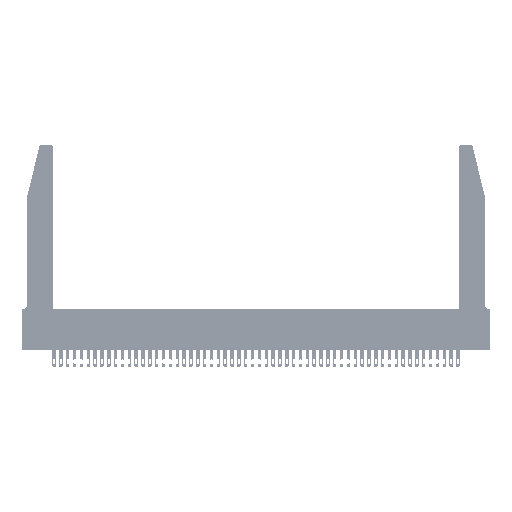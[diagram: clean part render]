
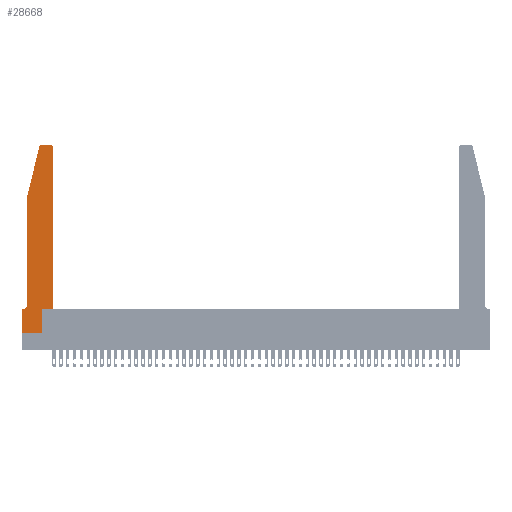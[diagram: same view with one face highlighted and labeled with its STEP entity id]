
A CAD part, top view. The second image highlights one B-rep face of the part: STEP entity #28668.
In plain terms, the highlighted planar face has unit normal (0, 0, 1).
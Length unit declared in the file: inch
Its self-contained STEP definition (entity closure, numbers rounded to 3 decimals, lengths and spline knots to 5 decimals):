
#95 = VERTEX_POINT ( 'NONE', #23272 ) ;
#1008 = EDGE_CURVE ( 'NONE', #95, #37372, #23729, .T. ) ;
#2778 = VERTEX_POINT ( 'NONE', #43819 ) ;
#3142 = LINE ( 'NONE', #47162, #42280 ) ;
#3506 = LINE ( 'NONE', #4900, #23275 ) ;
#3687 = CARTESIAN_POINT ( 'NONE',  ( 0.2605, 2.75, 0.37 ) ) ;
#4401 = AXIS2_PLACEMENT_3D ( 'NONE', #20127, #46738, #35255 ) ;
#4447 = EDGE_CURVE ( 'NONE', #40174, #19119, #18785, .T. ) ;
#4479 = DIRECTION ( 'NONE',  ( 0., 1., 0. ) ) ;
#4484 = DIRECTION ( 'NONE',  ( 0., -1., 0. ) ) ;
#4900 = CARTESIAN_POINT ( 'NONE',  ( 0.0755, 2., 0.37 ) ) ;
#5908 = ORIENTED_EDGE ( 'NONE', *, *, #28364, .T. ) ;
#6014 = CIRCLE ( 'NONE', #27575, 0.07 ) ;
#6198 = VERTEX_POINT ( 'NONE', #40890 ) ;
#6744 = LINE ( 'NONE', #16457, #46118 ) ;
#8923 = DIRECTION ( 'NONE',  ( -0.239, -0.971, 0. ) ) ;
#9158 = DIRECTION ( 'NONE',  ( 0., 1., 0. ) ) ;
#9476 = AXIS2_PLACEMENT_3D ( 'NONE', #13988, #40635, #25505 ) ;
#9744 = VECTOR ( 'NONE', #9769, 39.37008 ) ;
#9769 = DIRECTION ( 'NONE',  ( 1., 0., 0. ) ) ;
#10043 = DIRECTION ( 'NONE',  ( 0., 0., 1. ) ) ;
#10725 = CIRCLE ( 'NONE', #4401, 0.03 ) ;
#11917 = DIRECTION ( 'NONE',  ( 0., -1., 0. ) ) ;
#11953 = EDGE_CURVE ( 'NONE', #48616, #95, #40362, .T. ) ;
#11988 = VERTEX_POINT ( 'NONE', #24195 ) ;
#12738 = ORIENTED_EDGE ( 'NONE', *, *, #44541, .T. ) ;
#12746 = VECTOR ( 'NONE', #4479, 39.37008 ) ;
#13988 = CARTESIAN_POINT ( 'NONE',  ( 0.4205, 2.72, 0.37 ) ) ;
#14906 = CIRCLE ( 'NONE', #9476, 0.03 ) ;
#15025 = EDGE_CURVE ( 'NONE', #2778, #40174, #15081, .T. ) ;
#15081 = LINE ( 'NONE', #39755, #9744 ) ;
#15237 = DIRECTION ( 'NONE',  ( -1., 0., 0. ) ) ;
#15477 = ORIENTED_EDGE ( 'NONE', *, *, #37178, .T. ) ;
#16035 = CARTESIAN_POINT ( 'NONE',  ( 0.4505, 0.35, 0.37 ) ) ;
#16457 = CARTESIAN_POINT ( 'NONE',  ( 0.0755, 2., 0.37 ) ) ;
#17227 = ORIENTED_EDGE ( 'NONE', *, *, #22877, .T. ) ;
#17357 = AXIS2_PLACEMENT_3D ( 'NONE', #44189, #10043, #21411 ) ;
#18785 = LINE ( 'NONE', #16035, #12746 ) ;
#19119 = VERTEX_POINT ( 'NONE', #37972 ) ;
#19725 = CARTESIAN_POINT ( 'NONE',  ( 0.0755, 0.35, 0.37 ) ) ;
#20127 = CARTESIAN_POINT ( 'NONE',  ( 0.284, 2.72, 0.37 ) ) ;
#20181 = CARTESIAN_POINT ( 'NONE',  ( 0.4505, 0.35, 0.37 ) ) ;
#21346 = VECTOR ( 'NONE', #35187, 39.37008 ) ;
#21411 = DIRECTION ( 'NONE',  ( 1., 0., 0. ) ) ;
#21571 = ORIENTED_EDGE ( 'NONE', *, *, #15025, .T. ) ;
#21862 = EDGE_LOOP ( 'NONE', ( #5908, #17227, #15477, #31111, #12738, #35607, #35556, #39969, #30928, #21571, #33312, #34398 ) ) ;
#22164 = VERTEX_POINT ( 'NONE', #45468 ) ;
#22374 = CARTESIAN_POINT ( 'NONE',  ( 0., 0., 0.37 ) ) ;
#22877 = EDGE_CURVE ( 'NONE', #11988, #22164, #10725, .T. ) ;
#22930 = EDGE_CURVE ( 'NONE', #41983, #42928, #3506, .T. ) ;
#23272 = CARTESIAN_POINT ( 'NONE',  ( 0., 0.35, 0.37 ) ) ;
#23275 = VECTOR ( 'NONE', #11917, 39.37008 ) ;
#23671 = CARTESIAN_POINT ( 'NONE',  ( 0., 0., 0.37 ) ) ;
#23729 = LINE ( 'NONE', #23671, #30871 ) ;
#23917 = FACE_OUTER_BOUND ( 'NONE', #21862, .T. ) ;
#24195 = CARTESIAN_POINT ( 'NONE',  ( 0.284, 2.75, 0.37 ) ) ;
#25505 = DIRECTION ( 'NONE',  ( 1., 0., 0. ) ) ;
#25550 = PLANE ( 'NONE',  #17357 ) ;
#26196 = DIRECTION ( 'NONE',  ( 1., 0., 0. ) ) ;
#27547 = VECTOR ( 'NONE', #15237, 39.37008 ) ;
#27575 = AXIS2_PLACEMENT_3D ( 'NONE', #31802, #38970, #46809 ) ;
#28364 = EDGE_CURVE ( 'NONE', #6198, #11988, #47180, .T. ) ;
#28668 = ADVANCED_FACE ( 'NONE', ( #23917 ), #25550, .T. ) ;
#29450 = CARTESIAN_POINT ( 'NONE',  ( 0.0755, 0.42, 0.37 ) ) ;
#30328 = VERTEX_POINT ( 'NONE', #35889 ) ;
#30871 = VECTOR ( 'NONE', #4484, 39.37008 ) ;
#30928 = ORIENTED_EDGE ( 'NONE', *, *, #35849, .T. ) ;
#31111 = ORIENTED_EDGE ( 'NONE', *, *, #22930, .T. ) ;
#31802 = CARTESIAN_POINT ( 'NONE',  ( 0.0055, 0.42, 0.37 ) ) ;
#32052 = EDGE_CURVE ( 'NONE', #19119, #6198, #14906, .T. ) ;
#33233 = CARTESIAN_POINT ( 'NONE',  ( 0., 0., 0.37 ) ) ;
#33312 = ORIENTED_EDGE ( 'NONE', *, *, #4447, .T. ) ;
#34398 = ORIENTED_EDGE ( 'NONE', *, *, #32052, .T. ) ;
#34749 = LINE ( 'NONE', #22374, #46709 ) ;
#35187 = DIRECTION ( 'NONE',  ( -1., 0., 0. ) ) ;
#35255 = DIRECTION ( 'NONE',  ( 1., 0., 0. ) ) ;
#35556 = ORIENTED_EDGE ( 'NONE', *, *, #1008, .T. ) ;
#35607 = ORIENTED_EDGE ( 'NONE', *, *, #11953, .T. ) ;
#35849 = EDGE_CURVE ( 'NONE', #30328, #2778, #3142, .T. ) ;
#35889 = CARTESIAN_POINT ( 'NONE',  ( 0.2865, 0., 0.37 ) ) ;
#37178 = EDGE_CURVE ( 'NONE', #22164, #41983, #6744, .T. ) ;
#37372 = VERTEX_POINT ( 'NONE', #33233 ) ;
#37972 = CARTESIAN_POINT ( 'NONE',  ( 0.4505, 2.72, 0.37 ) ) ;
#38039 = EDGE_CURVE ( 'NONE', #37372, #30328, #34749, .T. ) ;
#38970 = DIRECTION ( 'NONE',  ( 0., 0., -1. ) ) ;
#39755 = CARTESIAN_POINT ( 'NONE',  ( 0.4505, 0.35, 0.37 ) ) ;
#39969 = ORIENTED_EDGE ( 'NONE', *, *, #38039, .T. ) ;
#40174 = VERTEX_POINT ( 'NONE', #20181 ) ;
#40333 = CARTESIAN_POINT ( 'NONE',  ( 0.0055, 0.35, 0.37 ) ) ;
#40362 = LINE ( 'NONE', #19725, #21346 ) ;
#40635 = DIRECTION ( 'NONE',  ( 0., 0., 1. ) ) ;
#40890 = CARTESIAN_POINT ( 'NONE',  ( 0.4205, 2.75, 0.37 ) ) ;
#41983 = VERTEX_POINT ( 'NONE', #42105 ) ;
#42105 = CARTESIAN_POINT ( 'NONE',  ( 0.0755, 2., 0.37 ) ) ;
#42280 = VECTOR ( 'NONE', #9158, 39.37008 ) ;
#42928 = VERTEX_POINT ( 'NONE', #29450 ) ;
#43819 = CARTESIAN_POINT ( 'NONE',  ( 0.2865, 0.35, 0.37 ) ) ;
#44189 = CARTESIAN_POINT ( 'NONE',  ( 0., 0.35, 0.37 ) ) ;
#44541 = EDGE_CURVE ( 'NONE', #42928, #48616, #6014, .T. ) ;
#45468 = CARTESIAN_POINT ( 'NONE',  ( 0.25487, 2.72718, 0.37 ) ) ;
#46118 = VECTOR ( 'NONE', #8923, 39.37008 ) ;
#46709 = VECTOR ( 'NONE', #26196, 39.37008 ) ;
#46738 = DIRECTION ( 'NONE',  ( 0., 0., 1. ) ) ;
#46809 = DIRECTION ( 'NONE',  ( -1., 0., 0. ) ) ;
#47162 = CARTESIAN_POINT ( 'NONE',  ( 0.2865, 0.35, 0.37 ) ) ;
#47180 = LINE ( 'NONE', #3687, #27547 ) ;
#48616 = VERTEX_POINT ( 'NONE', #40333 ) ;
